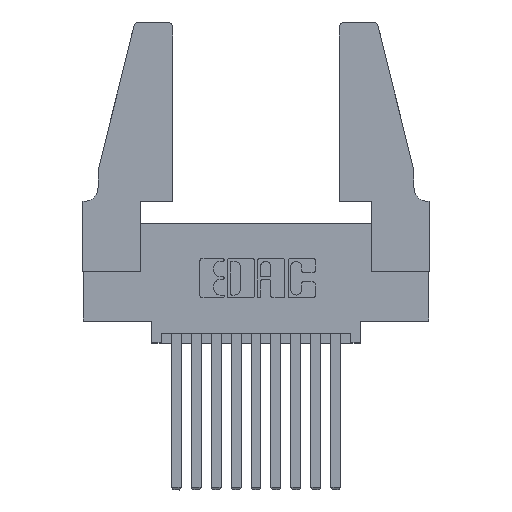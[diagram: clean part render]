
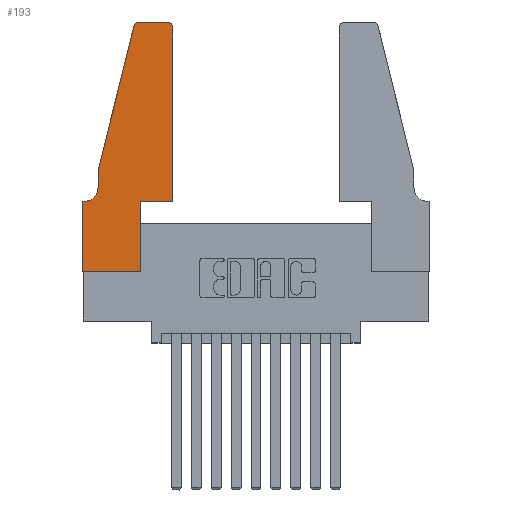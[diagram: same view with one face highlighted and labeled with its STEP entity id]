
A CAD part, top view. The second image highlights one B-rep face of the part: STEP entity #193.
In plain terms, the highlighted planar face has unit normal (0, 0, 1).
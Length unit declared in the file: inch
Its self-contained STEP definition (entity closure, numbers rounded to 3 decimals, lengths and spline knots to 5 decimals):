
#19 = VERTEX_POINT ( 'NONE', #1753 ) ;
#193 = ADVANCED_FACE ( 'NONE', ( #6088 ), #1356, .T. ) ;
#295 = EDGE_CURVE ( 'NONE', #10427, #19, #3440, .T. ) ;
#411 = LINE ( 'NONE', #12234, #8445 ) ;
#414 = DIRECTION ( 'NONE',  ( 0., 0., 1. ) ) ;
#558 = CARTESIAN_POINT ( 'NONE',  ( 0.25487, 1.22718, 0.37 ) ) ;
#594 = CARTESIAN_POINT ( 'NONE',  ( 0.2865, 0.35, 0.37 ) ) ;
#641 = CARTESIAN_POINT ( 'NONE',  ( 0.284, 1.22, 0.37 ) ) ;
#907 = EDGE_CURVE ( 'NONE', #3635, #1798, #13184, .T. ) ;
#1019 = VERTEX_POINT ( 'NONE', #5239 ) ;
#1356 = PLANE ( 'NONE',  #5049 ) ;
#1491 = VERTEX_POINT ( 'NONE', #13425 ) ;
#1496 = CARTESIAN_POINT ( 'NONE',  ( 0., 0., 0.37 ) ) ;
#1651 = ORIENTED_EDGE ( 'NONE', *, *, #3780, .T. ) ;
#1753 = CARTESIAN_POINT ( 'NONE',  ( 0., 0.35, 0.37 ) ) ;
#1798 = VERTEX_POINT ( 'NONE', #7391 ) ;
#2054 = ORIENTED_EDGE ( 'NONE', *, *, #7353, .T. ) ;
#2383 = DIRECTION ( 'NONE',  ( 0., -1., 0. ) ) ;
#2440 = DIRECTION ( 'NONE',  ( -1., 0., 0. ) ) ;
#2448 = DIRECTION ( 'NONE',  ( 0., 0., 1. ) ) ;
#2955 = VECTOR ( 'NONE', #2440, 39.37008 ) ;
#3440 = LINE ( 'NONE', #6773, #2955 ) ;
#3498 = DIRECTION ( 'NONE',  ( 1., 0., 0. ) ) ;
#3536 = EDGE_CURVE ( 'NONE', #9107, #8733, #8610, .T. ) ;
#3635 = VERTEX_POINT ( 'NONE', #9631 ) ;
#3641 = AXIS2_PLACEMENT_3D ( 'NONE', #641, #5875, #9037 ) ;
#3780 = EDGE_CURVE ( 'NONE', #19, #6762, #12094, .T. ) ;
#3922 = VECTOR ( 'NONE', #5564, 39.37008 ) ;
#3939 = CARTESIAN_POINT ( 'NONE',  ( 0.4505, 0.35, 0.37 ) ) ;
#4154 = LINE ( 'NONE', #4221, #10435 ) ;
#4221 = CARTESIAN_POINT ( 'NONE',  ( 0.2605, 1.25, 0.37 ) ) ;
#4269 = ORIENTED_EDGE ( 'NONE', *, *, #295, .T. ) ;
#4424 = VECTOR ( 'NONE', #12972, 39.37008 ) ;
#4581 = EDGE_CURVE ( 'NONE', #9868, #9107, #4154, .T. ) ;
#4586 = ORIENTED_EDGE ( 'NONE', *, *, #5997, .T. ) ;
#4592 = CARTESIAN_POINT ( 'NONE',  ( 0.4505, 0.35, 0.37 ) ) ;
#4668 = DIRECTION ( 'NONE',  ( 0., 0., -1. ) ) ;
#4756 = EDGE_CURVE ( 'NONE', #6110, #10427, #12885, .T. ) ;
#4823 = VECTOR ( 'NONE', #2383, 39.37008 ) ;
#5049 = AXIS2_PLACEMENT_3D ( 'NONE', #11905, #2448, #6553 ) ;
#5161 = ORIENTED_EDGE ( 'NONE', *, *, #5889, .T. ) ;
#5208 = EDGE_CURVE ( 'NONE', #1491, #6110, #9757, .T. ) ;
#5239 = CARTESIAN_POINT ( 'NONE',  ( 0.4505, 1.22, 0.37 ) ) ;
#5564 = DIRECTION ( 'NONE',  ( -0.239, -0.971, 0. ) ) ;
#5875 = DIRECTION ( 'NONE',  ( 0., 0., 1. ) ) ;
#5889 = EDGE_CURVE ( 'NONE', #13202, #1019, #12034, .T. ) ;
#5997 = EDGE_CURVE ( 'NONE', #6762, #3635, #11853, .T. ) ;
#6088 = FACE_OUTER_BOUND ( 'NONE', #7375, .T. ) ;
#6110 = VERTEX_POINT ( 'NONE', #11029 ) ;
#6553 = DIRECTION ( 'NONE',  ( 1., 0., 0. ) ) ;
#6560 = VECTOR ( 'NONE', #9068, 39.37008 ) ;
#6762 = VERTEX_POINT ( 'NONE', #1496 ) ;
#6770 = CARTESIAN_POINT ( 'NONE',  ( 0.4205, 1.22, 0.37 ) ) ;
#6773 = CARTESIAN_POINT ( 'NONE',  ( 0.0755, 0.35, 0.37 ) ) ;
#6875 = CIRCLE ( 'NONE', #7741, 0.03 ) ;
#6981 = ORIENTED_EDGE ( 'NONE', *, *, #4756, .T. ) ;
#7324 = EDGE_CURVE ( 'NONE', #1019, #9868, #6875, .T. ) ;
#7353 = EDGE_CURVE ( 'NONE', #8733, #1491, #13503, .T. ) ;
#7375 = EDGE_LOOP ( 'NONE', ( #10305, #9849, #2054, #11621, #6981, #4269, #1651, #4586, #7946, #9424, #5161, #10257 ) ) ;
#7391 = CARTESIAN_POINT ( 'NONE',  ( 0.2865, 0.35, 0.37 ) ) ;
#7649 = CARTESIAN_POINT ( 'NONE',  ( 0., 0., 0.37 ) ) ;
#7730 = DIRECTION ( 'NONE',  ( -1., 0., 0. ) ) ;
#7741 = AXIS2_PLACEMENT_3D ( 'NONE', #6770, #414, #3498 ) ;
#7742 = CARTESIAN_POINT ( 'NONE',  ( 0.0755, 0.5, 0.37 ) ) ;
#7946 = ORIENTED_EDGE ( 'NONE', *, *, #907, .T. ) ;
#8413 = VECTOR ( 'NONE', #12623, 39.37008 ) ;
#8445 = VECTOR ( 'NONE', #9155, 39.37008 ) ;
#8610 = CIRCLE ( 'NONE', #3641, 0.03 ) ;
#8733 = VERTEX_POINT ( 'NONE', #558 ) ;
#9008 = CARTESIAN_POINT ( 'NONE',  ( 0.4205, 1.25, 0.37 ) ) ;
#9037 = DIRECTION ( 'NONE',  ( 1., 0., 0. ) ) ;
#9068 = DIRECTION ( 'NONE',  ( 0., 1., 0. ) ) ;
#9107 = VERTEX_POINT ( 'NONE', #9112 ) ;
#9112 = CARTESIAN_POINT ( 'NONE',  ( 0.284, 1.25, 0.37 ) ) ;
#9155 = DIRECTION ( 'NONE',  ( 1., 0., 0. ) ) ;
#9253 = VECTOR ( 'NONE', #11117, 39.37008 ) ;
#9274 = CARTESIAN_POINT ( 'NONE',  ( 0.0055, 0.35, 0.37 ) ) ;
#9424 = ORIENTED_EDGE ( 'NONE', *, *, #11729, .T. ) ;
#9491 = CARTESIAN_POINT ( 'NONE',  ( 0.0755, 0.5, 0.37 ) ) ;
#9631 = CARTESIAN_POINT ( 'NONE',  ( 0.2865, 0., 0.37 ) ) ;
#9757 = LINE ( 'NONE', #9491, #8413 ) ;
#9849 = ORIENTED_EDGE ( 'NONE', *, *, #3536, .T. ) ;
#9868 = VERTEX_POINT ( 'NONE', #9008 ) ;
#9872 = CARTESIAN_POINT ( 'NONE',  ( 0.0055, 0.42, 0.37 ) ) ;
#10257 = ORIENTED_EDGE ( 'NONE', *, *, #7324, .T. ) ;
#10305 = ORIENTED_EDGE ( 'NONE', *, *, #4581, .T. ) ;
#10427 = VERTEX_POINT ( 'NONE', #9274 ) ;
#10435 = VECTOR ( 'NONE', #10590, 39.37008 ) ;
#10590 = DIRECTION ( 'NONE',  ( -1., 0., 0. ) ) ;
#11029 = CARTESIAN_POINT ( 'NONE',  ( 0.0755, 0.42, 0.37 ) ) ;
#11117 = DIRECTION ( 'NONE',  ( 0., 1., 0. ) ) ;
#11621 = ORIENTED_EDGE ( 'NONE', *, *, #5208, .T. ) ;
#11729 = EDGE_CURVE ( 'NONE', #1798, #13202, #411, .T. ) ;
#11845 = CARTESIAN_POINT ( 'NONE',  ( 0., 0., 0.37 ) ) ;
#11853 = LINE ( 'NONE', #11845, #4424 ) ;
#11905 = CARTESIAN_POINT ( 'NONE',  ( 0., 0.35, 0.37 ) ) ;
#12034 = LINE ( 'NONE', #4592, #9253 ) ;
#12094 = LINE ( 'NONE', #7649, #4823 ) ;
#12234 = CARTESIAN_POINT ( 'NONE',  ( 0.4505, 0.35, 0.37 ) ) ;
#12623 = DIRECTION ( 'NONE',  ( 0., -1., 0. ) ) ;
#12885 = CIRCLE ( 'NONE', #13308, 0.07 ) ;
#12972 = DIRECTION ( 'NONE',  ( 1., 0., 0. ) ) ;
#13184 = LINE ( 'NONE', #594, #6560 ) ;
#13202 = VERTEX_POINT ( 'NONE', #3939 ) ;
#13308 = AXIS2_PLACEMENT_3D ( 'NONE', #9872, #4668, #7730 ) ;
#13425 = CARTESIAN_POINT ( 'NONE',  ( 0.0755, 0.5, 0.37 ) ) ;
#13503 = LINE ( 'NONE', #7742, #3922 ) ;
